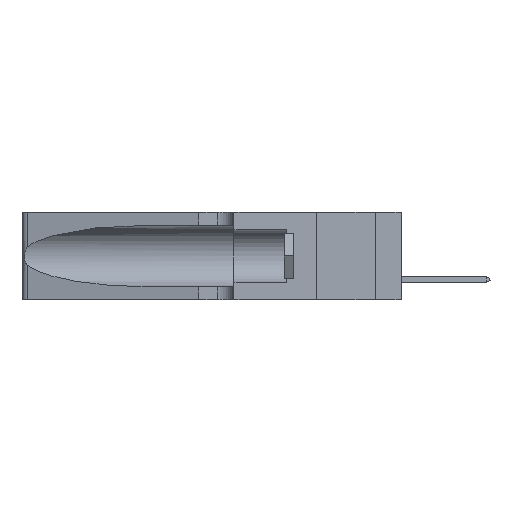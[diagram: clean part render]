
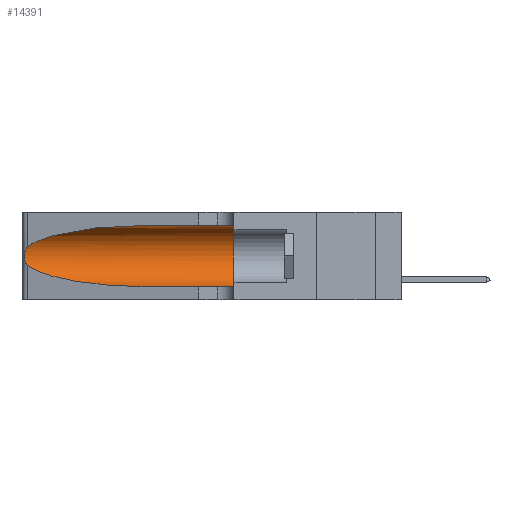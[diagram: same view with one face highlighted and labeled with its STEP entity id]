
A CAD part, left-side view. The second image highlights one B-rep face of the part: STEP entity #14391.
In plain terms, the highlighted cylindrical face has radius 3.308 mm (diameter 6.617 mm), a partial arc.
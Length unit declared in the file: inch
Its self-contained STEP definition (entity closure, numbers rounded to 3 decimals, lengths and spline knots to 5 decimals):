
#485 = LINE ( 'NONE', #5632, #22524 ) ;
#1349 = CARTESIAN_POINT ( 'NONE',  ( 0.25789, 1.23486, 0.15765 ) ) ;
#2125 = DIRECTION ( 'NONE',  ( 0., 0., -1. ) ) ;
#2252 = CARTESIAN_POINT ( 'NONE',  ( 0.1305, 1.61858, 0.185 ) ) ;
#4523 = CARTESIAN_POINT ( 'NONE',  ( 0.26017, 1.23833, 0.17102 ) ) ;
#5170 = CARTESIAN_POINT ( 'NONE',  ( 0.18966, 0.96281, 0.31525 ) ) ;
#5632 = CARTESIAN_POINT ( 'NONE',  ( 0.1305, 1.61858, 0.31525 ) ) ;
#6473 = EDGE_CURVE ( 'NONE', #34112, #25380, #485, .T. ) ;
#8186 = CARTESIAN_POINT ( 'NONE',  ( 0.1305, 0.35, 0.185 ) ) ;
#8276 = ORIENTED_EDGE ( 'NONE', *, *, #12329, .F. ) ;
#9232 = CIRCLE ( 'NONE', #30238, 0.13025 ) ;
#9300 = DIRECTION ( 'NONE',  ( 0., -1., 0. ) ) ;
#10117 = ORIENTED_EDGE ( 'NONE', *, *, #24173, .T. ) ;
#10210 = ORIENTED_EDGE ( 'NONE', *, *, #30184, .T. ) ;
#10442 = CARTESIAN_POINT ( 'NONE',  ( 0.25487, 1.22718, 0.14631 ) ) ;
#10839 = CARTESIAN_POINT ( 'NONE',  ( 0.25639, 1.23186, 0.15144 ) ) ;
#10990 = CARTESIAN_POINT ( 'NONE',  ( 0.25856, 1.23593, 0.16098 ) ) ;
#11139 = CARTESIAN_POINT ( 'NONE',  ( 0.26018, 1.23835, 0.19895 ) ) ;
#11539 = DIRECTION ( 'NONE',  ( 0., 0., 1. ) ) ;
#12329 = EDGE_CURVE ( 'NONE', #25380, #24289, #9232, .T. ) ;
#13483 = EDGE_LOOP ( 'NONE', ( #25297, #10117, #10210, #38797, #8276, #14623 ) ) ;
#14087 = CARTESIAN_POINT ( 'NONE',  ( 0.2373, 1.15595, 0.08982 ) ) ;
#14391 = ADVANCED_FACE ( 'NONE', ( #15034 ), #19054, .F. ) ;
#14623 = ORIENTED_EDGE ( 'NONE', *, *, #6473, .F. ) ;
#15034 = FACE_OUTER_BOUND ( 'NONE', #13483, .T. ) ;
#16587 = CARTESIAN_POINT ( 'NONE',  ( 0.1305, 0.72297, 0.05475 ) ) ;
#17210 = EDGE_CURVE ( 'NONE', #34112, #19047, #22430, .T. ) ;
#17558 = DIRECTION ( 'NONE',  ( 0., 1., 0. ) ) ;
#18261 = DIRECTION ( 'NONE',  ( 0., -1., 0. ) ) ;
#19047 = VERTEX_POINT ( 'NONE', #24107 ) ;
#19054 = CYLINDRICAL_SURFACE ( 'NONE', #20901, 0.13025 ) ;
#19329 =( BOUNDED_CURVE ( )  B_SPLINE_CURVE ( 3, ( #10442, #14087, #23341, #23774 ),
 .UNSPECIFIED., .F., .T. ) 
 B_SPLINE_CURVE_WITH_KNOTS ( ( 4, 4 ),
 ( 3.44316, 4.71239 ),
 .UNSPECIFIED. ) 
 CURVE ( )  GEOMETRIC_REPRESENTATION_ITEM ( )  RATIONAL_B_SPLINE_CURVE ( ( 1., 0.87, 0.87, 1. ) ) 
 REPRESENTATION_ITEM ( '' )  );
#19376 = CARTESIAN_POINT ( 'NONE',  ( 0.25787, 1.23484, 0.2124 ) ) ;
#19768 = CARTESIAN_POINT ( 'NONE',  ( 0.1305, 0.35, 0.31525 ) ) ;
#19953 = CARTESIAN_POINT ( 'NONE',  ( 0.1305, 0.72297, 0.31525 ) ) ;
#20512 = CARTESIAN_POINT ( 'NONE',  ( 0.26075, 1.23896, 0.178 ) ) ;
#20901 = AXIS2_PLACEMENT_3D ( 'NONE', #2252, #36868, #2125 ) ;
#21651 = CARTESIAN_POINT ( 'NONE',  ( 0.1305, 1.61858, 0.05475 ) ) ;
#21954 = CARTESIAN_POINT ( 'NONE',  ( 0.25487, 1.22718, 0.22369 ) ) ;
#22430 =( BOUNDED_CURVE ( )  B_SPLINE_CURVE ( 3, ( #27288, #5170, #30469, #33685 ),
 .UNSPECIFIED., .F., .F. ) 
 B_SPLINE_CURVE_WITH_KNOTS ( ( 4, 4 ),
 ( 1.5708, 2.84003 ),
 .UNSPECIFIED. ) 
 CURVE ( )  GEOMETRIC_REPRESENTATION_ITEM ( )  RATIONAL_B_SPLINE_CURVE ( ( 1., 0.87, 0.87, 1. ) ) 
 REPRESENTATION_ITEM ( '' )  );
#22524 = VECTOR ( 'NONE', #18261, 39.37008 ) ;
#23341 = CARTESIAN_POINT ( 'NONE',  ( 0.18966, 0.96281, 0.05475 ) ) ;
#23568 = VERTEX_POINT ( 'NONE', #26561 ) ;
#23774 = CARTESIAN_POINT ( 'NONE',  ( 0.1305, 0.72297, 0.05475 ) ) ;
#24107 = CARTESIAN_POINT ( 'NONE',  ( 0.25487, 1.22718, 0.22369 ) ) ;
#24173 = EDGE_CURVE ( 'NONE', #19047, #23568, #26763, .T. ) ;
#24289 = VERTEX_POINT ( 'NONE', #30272 ) ;
#25297 = ORIENTED_EDGE ( 'NONE', *, *, #17210, .T. ) ;
#25380 = VERTEX_POINT ( 'NONE', #19768 ) ;
#26561 = CARTESIAN_POINT ( 'NONE',  ( 0.25487, 1.22718, 0.14631 ) ) ;
#26573 = EDGE_CURVE ( 'NONE', #40943, #24289, #29026, .T. ) ;
#26763 = B_SPLINE_CURVE_WITH_KNOTS ( 'NONE', 3,
 ( #21954, #34342, #32176, #19376, #39616, #11139, #36535, #20512, #4523, #10990, #1349, #10839, #26925, #33037 ),
 .UNSPECIFIED., .F., .F.,
 ( 4, 2, 2, 2, 2, 2, 4 ),
 ( 0., 0.00027, 0.00053, 0.00107, 0.0016, 0.00187, 0.00214 ),
 .UNSPECIFIED. ) ;
#26925 = CARTESIAN_POINT ( 'NONE',  ( 0.25555, 1.22993, 0.14849 ) ) ;
#27079 = VECTOR ( 'NONE', #9300, 39.37008 ) ;
#27288 = CARTESIAN_POINT ( 'NONE',  ( 0.1305, 0.72297, 0.31525 ) ) ;
#29026 = LINE ( 'NONE', #21651, #27079 ) ;
#30184 = EDGE_CURVE ( 'NONE', #23568, #40943, #19329, .T. ) ;
#30238 = AXIS2_PLACEMENT_3D ( 'NONE', #8186, #17558, #11539 ) ;
#30272 = CARTESIAN_POINT ( 'NONE',  ( 0.1305, 0.35, 0.05475 ) ) ;
#30469 = CARTESIAN_POINT ( 'NONE',  ( 0.2373, 1.15595, 0.28018 ) ) ;
#32176 = CARTESIAN_POINT ( 'NONE',  ( 0.25639, 1.23184, 0.21858 ) ) ;
#33037 = CARTESIAN_POINT ( 'NONE',  ( 0.25487, 1.22718, 0.14631 ) ) ;
#33685 = CARTESIAN_POINT ( 'NONE',  ( 0.25487, 1.22718, 0.22369 ) ) ;
#34112 = VERTEX_POINT ( 'NONE', #19953 ) ;
#34342 = CARTESIAN_POINT ( 'NONE',  ( 0.25555, 1.22994, 0.2215 ) ) ;
#36535 = CARTESIAN_POINT ( 'NONE',  ( 0.26075, 1.23896, 0.19203 ) ) ;
#36868 = DIRECTION ( 'NONE',  ( 0., -1., 0. ) ) ;
#38797 = ORIENTED_EDGE ( 'NONE', *, *, #26573, .T. ) ;
#39616 = CARTESIAN_POINT ( 'NONE',  ( 0.25854, 1.2359, 0.20912 ) ) ;
#40943 = VERTEX_POINT ( 'NONE', #16587 ) ;
